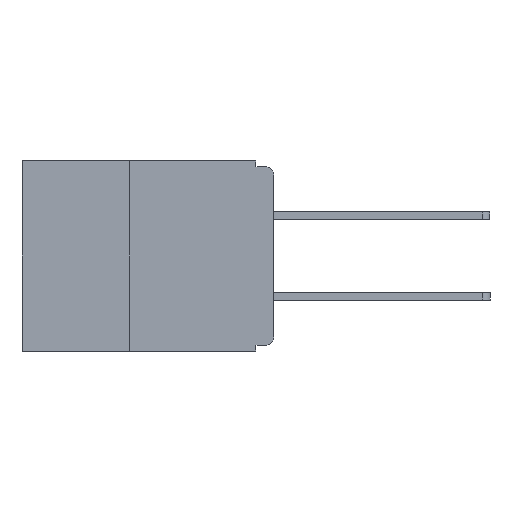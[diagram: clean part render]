
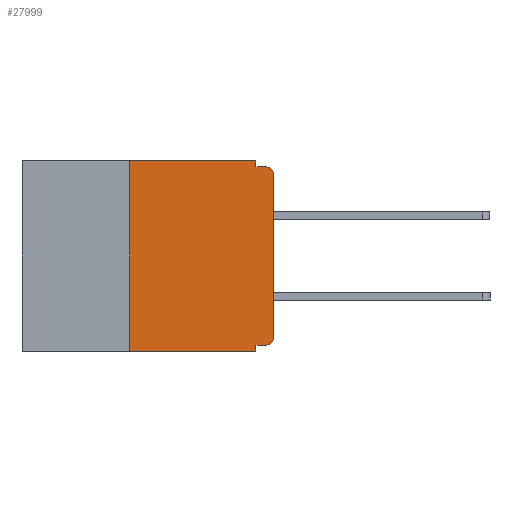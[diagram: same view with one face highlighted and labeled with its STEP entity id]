
A CAD part, left-side view. The second image highlights one B-rep face of the part: STEP entity #27999.
In plain terms, the highlighted planar face has unit normal (-1, 0, 0).
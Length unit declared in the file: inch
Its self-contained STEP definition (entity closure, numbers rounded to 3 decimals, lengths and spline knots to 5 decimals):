
#90 = CARTESIAN_POINT ( 'NONE',  ( 0., 0.015, -0.305 ) ) ;
#1253 = CARTESIAN_POINT ( 'NONE',  ( 0., 0.437, 0. ) ) ;
#2640 = DIRECTION ( 'NONE',  ( 0., 0., -1. ) ) ;
#2785 = CARTESIAN_POINT ( 'NONE',  ( 0., 0.015, -0.025 ) ) ;
#3820 = CARTESIAN_POINT ( 'NONE',  ( 0., 0., 0. ) ) ;
#3983 = CIRCLE ( 'NONE', #5166, 0.015 ) ;
#4214 = DIRECTION ( 'NONE',  ( 0., -1., 0. ) ) ;
#5123 = AXIS2_PLACEMENT_3D ( 'NONE', #2785, #20148, #5323 ) ;
#5166 = AXIS2_PLACEMENT_3D ( 'NONE', #90, #17548, #2640 ) ;
#5323 = DIRECTION ( 'NONE',  ( 0., 0., -1. ) ) ;
#5448 = VERTEX_POINT ( 'NONE', #7372 ) ;
#5971 = LINE ( 'NONE', #11307, #31222 ) ;
#6168 = CARTESIAN_POINT ( 'NONE',  ( 0., 0.015, -0.32 ) ) ;
#6268 = EDGE_CURVE ( 'NONE', #30283, #23210, #28094, .T. ) ;
#6377 = ORIENTED_EDGE ( 'NONE', *, *, #26275, .T. ) ;
#7243 = LINE ( 'NONE', #11585, #21211 ) ;
#7315 = CARTESIAN_POINT ( 'NONE',  ( 0., 0.031, -0.01 ) ) ;
#7372 = CARTESIAN_POINT ( 'NONE',  ( 0., 0., -0.025 ) ) ;
#7555 = DIRECTION ( 'NONE',  ( 1., 0., 0. ) ) ;
#7843 = CARTESIAN_POINT ( 'NONE',  ( 0., 0.031, -0.32 ) ) ;
#7951 = EDGE_CURVE ( 'NONE', #23210, #11913, #25943, .T. ) ;
#8945 = DIRECTION ( 'NONE',  ( 0., -1., 0. ) ) ;
#9258 = CARTESIAN_POINT ( 'NONE',  ( 0., 0.25, -0.33 ) ) ;
#9321 = LINE ( 'NONE', #3820, #15179 ) ;
#9649 = VERTEX_POINT ( 'NONE', #6168 ) ;
#9777 = ORIENTED_EDGE ( 'NONE', *, *, #23979, .T. ) ;
#10053 = VECTOR ( 'NONE', #29214, 39.37008 ) ;
#10979 = CIRCLE ( 'NONE', #5123, 0.015 ) ;
#11307 = CARTESIAN_POINT ( 'NONE',  ( 0., 0.031, -0.33 ) ) ;
#11355 = VECTOR ( 'NONE', #15785, 39.37008 ) ;
#11585 = CARTESIAN_POINT ( 'NONE',  ( 0., 0.437, -0.33 ) ) ;
#11783 = ORIENTED_EDGE ( 'NONE', *, *, #29376, .T. ) ;
#11913 = VERTEX_POINT ( 'NONE', #28210 ) ;
#12129 = CARTESIAN_POINT ( 'NONE',  ( 0., 0.031, 0. ) ) ;
#12889 = LINE ( 'NONE', #13291, #11355 ) ;
#13291 = CARTESIAN_POINT ( 'NONE',  ( 0., 0.25, -0.33 ) ) ;
#15179 = VECTOR ( 'NONE', #16299, 39.37008 ) ;
#15317 = CARTESIAN_POINT ( 'NONE',  ( 0., 0.031, 0. ) ) ;
#15686 = VECTOR ( 'NONE', #23570, 39.37008 ) ;
#15785 = DIRECTION ( 'NONE',  ( 0., 0., 1. ) ) ;
#16299 = DIRECTION ( 'NONE',  ( 0., 0., 1. ) ) ;
#16815 = VERTEX_POINT ( 'NONE', #23456 ) ;
#16857 = EDGE_CURVE ( 'NONE', #30555, #30283, #17220, .T. ) ;
#16886 = CARTESIAN_POINT ( 'NONE',  ( 0., 0., -0.32 ) ) ;
#17194 = ORIENTED_EDGE ( 'NONE', *, *, #7951, .F. ) ;
#17220 = LINE ( 'NONE', #1253, #15686 ) ;
#17548 = DIRECTION ( 'NONE',  ( -1., 0., 0. ) ) ;
#17989 = ORIENTED_EDGE ( 'NONE', *, *, #24906, .F. ) ;
#18716 = VECTOR ( 'NONE', #4214, 39.37008 ) ;
#19096 = EDGE_CURVE ( 'NONE', #16815, #5448, #9321, .T. ) ;
#19356 = DIRECTION ( 'NONE',  ( 0., 1., 0. ) ) ;
#19914 = PLANE ( 'NONE',  #27851 ) ;
#20148 = DIRECTION ( 'NONE',  ( -1., 0., 0. ) ) ;
#20978 = LINE ( 'NONE', #16886, #26626 ) ;
#21070 = ORIENTED_EDGE ( 'NONE', *, *, #6268, .F. ) ;
#21211 = VECTOR ( 'NONE', #8945, 39.37008 ) ;
#22051 = FACE_OUTER_BOUND ( 'NONE', #29628, .T. ) ;
#22374 = CARTESIAN_POINT ( 'NONE',  ( 0., 0.437, 0. ) ) ;
#22811 = EDGE_CURVE ( 'NONE', #26844, #29794, #5971, .T. ) ;
#23210 = VERTEX_POINT ( 'NONE', #7315 ) ;
#23456 = CARTESIAN_POINT ( 'NONE',  ( 0., 0., -0.305 ) ) ;
#23465 = EDGE_CURVE ( 'NONE', #24869, #30555, #12889, .T. ) ;
#23570 = DIRECTION ( 'NONE',  ( 0., -1., 0. ) ) ;
#23680 = DIRECTION ( 'NONE',  ( 0., 0., -1. ) ) ;
#23979 = EDGE_CURVE ( 'NONE', #5448, #11913, #10979, .T. ) ;
#24807 = DIRECTION ( 'NONE',  ( 0., 0., -1. ) ) ;
#24869 = VERTEX_POINT ( 'NONE', #9258 ) ;
#24906 = EDGE_CURVE ( 'NONE', #9649, #26844, #20978, .T. ) ;
#25622 = CARTESIAN_POINT ( 'NONE',  ( 0., 0.031, -0.33 ) ) ;
#25943 = LINE ( 'NONE', #28706, #18716 ) ;
#26275 = EDGE_CURVE ( 'NONE', #9649, #16815, #3983, .T. ) ;
#26626 = VECTOR ( 'NONE', #19356, 39.37008 ) ;
#26844 = VERTEX_POINT ( 'NONE', #7843 ) ;
#27851 = AXIS2_PLACEMENT_3D ( 'NONE', #22374, #7555, #24807 ) ;
#27999 = ADVANCED_FACE ( 'NONE', ( #22051 ), #19914, .F. ) ;
#28094 = LINE ( 'NONE', #12129, #10053 ) ;
#28210 = CARTESIAN_POINT ( 'NONE',  ( 0., 0.015, -0.01 ) ) ;
#28593 = ORIENTED_EDGE ( 'NONE', *, *, #19096, .T. ) ;
#28615 = CARTESIAN_POINT ( 'NONE',  ( 0., 0.25, 0. ) ) ;
#28625 = ORIENTED_EDGE ( 'NONE', *, *, #22811, .F. ) ;
#28706 = CARTESIAN_POINT ( 'NONE',  ( 0., 0., -0.01 ) ) ;
#29214 = DIRECTION ( 'NONE',  ( 0., 0., -1. ) ) ;
#29376 = EDGE_CURVE ( 'NONE', #24869, #29794, #7243, .T. ) ;
#29628 = EDGE_LOOP ( 'NONE', ( #28593, #9777, #17194, #21070, #29744, #30488, #11783, #28625, #17989, #6377 ) ) ;
#29744 = ORIENTED_EDGE ( 'NONE', *, *, #16857, .F. ) ;
#29794 = VERTEX_POINT ( 'NONE', #25622 ) ;
#30283 = VERTEX_POINT ( 'NONE', #15317 ) ;
#30488 = ORIENTED_EDGE ( 'NONE', *, *, #23465, .F. ) ;
#30555 = VERTEX_POINT ( 'NONE', #28615 ) ;
#31222 = VECTOR ( 'NONE', #23680, 39.37008 ) ;
